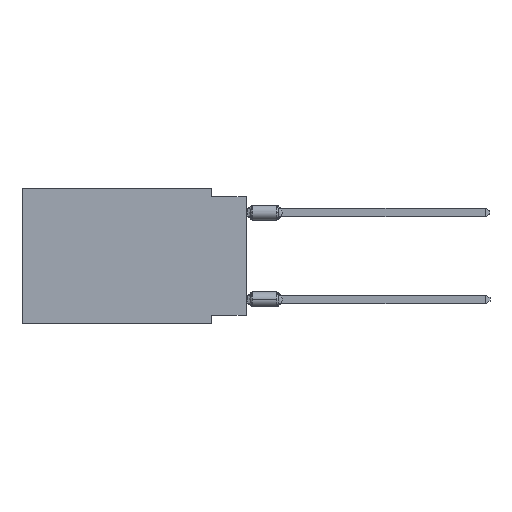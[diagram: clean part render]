
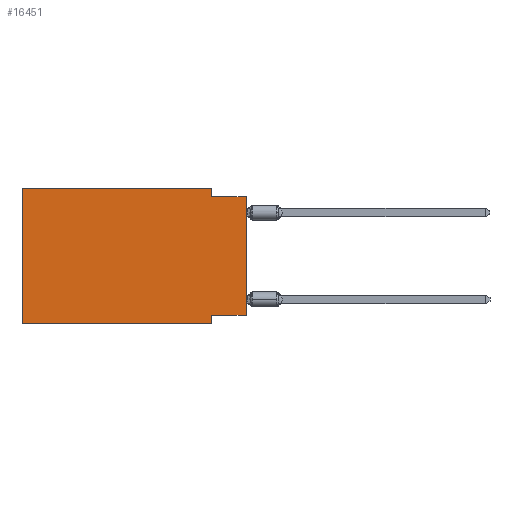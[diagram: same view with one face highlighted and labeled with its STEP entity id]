
A CAD part, left-side view. The second image highlights one B-rep face of the part: STEP entity #16451.
In plain terms, the highlighted planar face has unit normal (-1, 0, 0).
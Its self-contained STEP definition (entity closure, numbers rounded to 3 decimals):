
#132 = ORIENTED_EDGE ( 'NONE', *, *, #15119, .F. ) ;
#153 = CARTESIAN_POINT ( 'NONE',  ( 0., 0., 0. ) ) ;
#1259 = VECTOR ( 'NONE', #2261, 1000. ) ;
#1393 = CARTESIAN_POINT ( 'NONE',  ( 0., 16.383, 0. ) ) ;
#2133 = DIRECTION ( 'NONE',  ( 0., 0., 1. ) ) ;
#2146 = ORIENTED_EDGE ( 'NONE', *, *, #6252, .T. ) ;
#2261 = DIRECTION ( 'NONE',  ( 0., 0., -1. ) ) ;
#2382 = ORIENTED_EDGE ( 'NONE', *, *, #17018, .F. ) ;
#2389 = VECTOR ( 'NONE', #2133, 1000. ) ;
#2541 = CARTESIAN_POINT ( 'NONE',  ( 0., 0., -9.271 ) ) ;
#2795 = LINE ( 'NONE', #2541, #6500 ) ;
#3544 = LINE ( 'NONE', #23873, #5455 ) ;
#3564 = VERTEX_POINT ( 'NONE', #1393 ) ;
#4567 = CARTESIAN_POINT ( 'NONE',  ( 0., 16.383, -9.906 ) ) ;
#4636 = VECTOR ( 'NONE', #21763, 1000. ) ;
#5455 = VECTOR ( 'NONE', #9273, 1000. ) ;
#5509 = LINE ( 'NONE', #153, #21088 ) ;
#5547 = CARTESIAN_POINT ( 'NONE',  ( 0., 2.54, 0. ) ) ;
#5733 = LINE ( 'NONE', #13208, #5769 ) ;
#5769 = VECTOR ( 'NONE', #21161, 1000. ) ;
#6252 = EDGE_CURVE ( 'NONE', #14644, #19402, #3544, .T. ) ;
#6500 = VECTOR ( 'NONE', #10683, 1000. ) ;
#7122 = EDGE_CURVE ( 'NONE', #14644, #3564, #11164, .T. ) ;
#7819 = CARTESIAN_POINT ( 'NONE',  ( 0., 2.54, -9.271 ) ) ;
#8165 = CARTESIAN_POINT ( 'NONE',  ( 0., 0., -0.635 ) ) ;
#8195 = AXIS2_PLACEMENT_3D ( 'NONE', #24064, #14537, #24180 ) ;
#8358 = EDGE_CURVE ( 'NONE', #17312, #17723, #20745, .T. ) ;
#9182 = DIRECTION ( 'NONE',  ( 0., 0., 1. ) ) ;
#9273 = DIRECTION ( 'NONE',  ( 0., -1., 0. ) ) ;
#10683 = DIRECTION ( 'NONE',  ( 0., 1., 0. ) ) ;
#10714 = PLANE ( 'NONE',  #8195 ) ;
#11164 = LINE ( 'NONE', #22811, #2389 ) ;
#11508 = ORIENTED_EDGE ( 'NONE', *, *, #22395, .F. ) ;
#12119 = EDGE_LOOP ( 'NONE', ( #19985, #2382, #13718, #11508, #12903, #2146, #18401, #132 ) ) ;
#12209 = LINE ( 'NONE', #12327, #4636 ) ;
#12327 = CARTESIAN_POINT ( 'NONE',  ( 0., 16.383, 0. ) ) ;
#12446 = CARTESIAN_POINT ( 'NONE',  ( 0., 2.54, -9.906 ) ) ;
#12903 = ORIENTED_EDGE ( 'NONE', *, *, #7122, .F. ) ;
#13208 = CARTESIAN_POINT ( 'NONE',  ( 0., 2.54, -9.906 ) ) ;
#13525 = CARTESIAN_POINT ( 'NONE',  ( 0., 2.54, 0. ) ) ;
#13718 = ORIENTED_EDGE ( 'NONE', *, *, #8358, .F. ) ;
#14167 = DIRECTION ( 'NONE',  ( 0., -1., 0. ) ) ;
#14466 = CARTESIAN_POINT ( 'NONE',  ( 0., 0., -9.271 ) ) ;
#14537 = DIRECTION ( 'NONE',  ( 1., 0., 0. ) ) ;
#14644 = VERTEX_POINT ( 'NONE', #4567 ) ;
#14649 = FACE_OUTER_BOUND ( 'NONE', #12119, .T. ) ;
#15119 = EDGE_CURVE ( 'NONE', #23248, #23580, #2795, .T. ) ;
#15986 = VECTOR ( 'NONE', #14167, 1000. ) ;
#16451 = ADVANCED_FACE ( 'NONE', ( #14649 ), #10714, .F. ) ;
#17018 = EDGE_CURVE ( 'NONE', #17723, #18047, #17490, .T. ) ;
#17312 = VERTEX_POINT ( 'NONE', #13525 ) ;
#17490 = LINE ( 'NONE', #8165, #15986 ) ;
#17723 = VERTEX_POINT ( 'NONE', #21172 ) ;
#18047 = VERTEX_POINT ( 'NONE', #21026 ) ;
#18401 = ORIENTED_EDGE ( 'NONE', *, *, #23485, .F. ) ;
#19402 = VERTEX_POINT ( 'NONE', #12446 ) ;
#19985 = ORIENTED_EDGE ( 'NONE', *, *, #21744, .T. ) ;
#20745 = LINE ( 'NONE', #5547, #1259 ) ;
#21026 = CARTESIAN_POINT ( 'NONE',  ( 0., 0., -0.635 ) ) ;
#21088 = VECTOR ( 'NONE', #9182, 1000. ) ;
#21161 = DIRECTION ( 'NONE',  ( 0., 0., -1. ) ) ;
#21172 = CARTESIAN_POINT ( 'NONE',  ( 0., 2.54, -0.635 ) ) ;
#21744 = EDGE_CURVE ( 'NONE', #23248, #18047, #5509, .T. ) ;
#21763 = DIRECTION ( 'NONE',  ( 0., -1., 0. ) ) ;
#22395 = EDGE_CURVE ( 'NONE', #3564, #17312, #12209, .T. ) ;
#22811 = CARTESIAN_POINT ( 'NONE',  ( 0., 16.383, 0. ) ) ;
#23248 = VERTEX_POINT ( 'NONE', #14466 ) ;
#23485 = EDGE_CURVE ( 'NONE', #23580, #19402, #5733, .T. ) ;
#23580 = VERTEX_POINT ( 'NONE', #7819 ) ;
#23873 = CARTESIAN_POINT ( 'NONE',  ( 0., 16.383, -9.906 ) ) ;
#24064 = CARTESIAN_POINT ( 'NONE',  ( 0., 16.383, 0. ) ) ;
#24180 = DIRECTION ( 'NONE',  ( 0., 0., -1. ) ) ;
